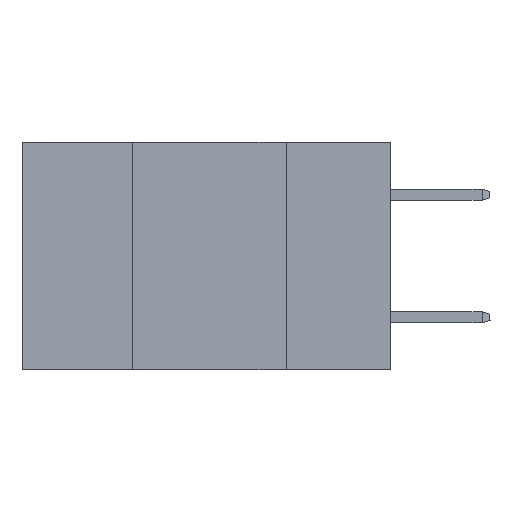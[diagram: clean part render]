
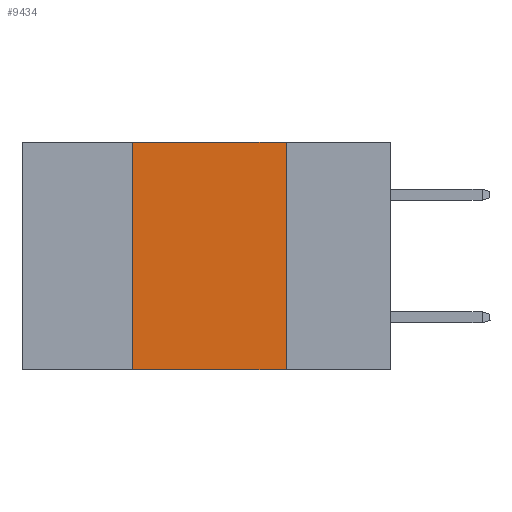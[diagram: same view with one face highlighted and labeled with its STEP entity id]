
A CAD part, left-side view. The second image highlights one B-rep face of the part: STEP entity #9434.
In plain terms, the highlighted planar face has unit normal (-1, 0, 0).
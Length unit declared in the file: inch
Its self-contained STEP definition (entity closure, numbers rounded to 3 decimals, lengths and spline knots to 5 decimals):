
#2066 = DIRECTION ( 'NONE',  ( 0., 0., -1. ) ) ;
#2339 = DIRECTION ( 'NONE',  ( 0., 0., 1. ) ) ;
#3312 = VECTOR ( 'NONE', #12593, 39.37008 ) ;
#4513 = CARTESIAN_POINT ( 'NONE',  ( 0., 0.42, -0.37 ) ) ;
#4653 = VERTEX_POINT ( 'NONE', #4513 ) ;
#4867 = CARTESIAN_POINT ( 'NONE',  ( 0., 0.17, 0. ) ) ;
#5146 = VERTEX_POINT ( 'NONE', #15281 ) ;
#5722 = DIRECTION ( 'NONE',  ( 0., -1., 0. ) ) ;
#5982 = LINE ( 'NONE', #27643, #36046 ) ;
#6003 = ORIENTED_EDGE ( 'NONE', *, *, #8970, .F. ) ;
#6198 = CARTESIAN_POINT ( 'NONE',  ( 0., 0.17, -0.37 ) ) ;
#6625 = VERTEX_POINT ( 'NONE', #15080 ) ;
#7380 = LINE ( 'NONE', #35424, #14434 ) ;
#7437 = AXIS2_PLACEMENT_3D ( 'NONE', #35588, #21869, #2066 ) ;
#8970 = EDGE_CURVE ( 'NONE', #6625, #31589, #18773, .T. ) ;
#9434 = ADVANCED_FACE ( 'NONE', ( #27364 ), #27190, .F. ) ;
#10148 = EDGE_LOOP ( 'NONE', ( #6003, #30099, #22833, #24137 ) ) ;
#12593 = DIRECTION ( 'NONE',  ( 0., 0., -1. ) ) ;
#13621 = CARTESIAN_POINT ( 'NONE',  ( 0., 0.6, 0. ) ) ;
#14097 = VECTOR ( 'NONE', #5722, 39.37008 ) ;
#14434 = VECTOR ( 'NONE', #29763, 39.37008 ) ;
#15080 = CARTESIAN_POINT ( 'NONE',  ( 0., 0.17, 0. ) ) ;
#15281 = CARTESIAN_POINT ( 'NONE',  ( 0., 0.42, 0. ) ) ;
#16264 = EDGE_CURVE ( 'NONE', #5146, #6625, #27929, .T. ) ;
#18773 = LINE ( 'NONE', #4867, #3312 ) ;
#21869 = DIRECTION ( 'NONE',  ( 1., 0., 0. ) ) ;
#22833 = ORIENTED_EDGE ( 'NONE', *, *, #33084, .F. ) ;
#24137 = ORIENTED_EDGE ( 'NONE', *, *, #32155, .T. ) ;
#27190 = PLANE ( 'NONE',  #7437 ) ;
#27364 = FACE_OUTER_BOUND ( 'NONE', #10148, .T. ) ;
#27643 = CARTESIAN_POINT ( 'NONE',  ( 0., 0.42, 0. ) ) ;
#27929 = LINE ( 'NONE', #13621, #14097 ) ;
#29763 = DIRECTION ( 'NONE',  ( 0., -1., 0. ) ) ;
#30099 = ORIENTED_EDGE ( 'NONE', *, *, #16264, .F. ) ;
#31589 = VERTEX_POINT ( 'NONE', #6198 ) ;
#32155 = EDGE_CURVE ( 'NONE', #4653, #31589, #7380, .T. ) ;
#33084 = EDGE_CURVE ( 'NONE', #4653, #5146, #5982, .T. ) ;
#35424 = CARTESIAN_POINT ( 'NONE',  ( 0., 0.6, -0.37 ) ) ;
#35588 = CARTESIAN_POINT ( 'NONE',  ( 0., 0.6, 0. ) ) ;
#36046 = VECTOR ( 'NONE', #2339, 39.37008 ) ;
